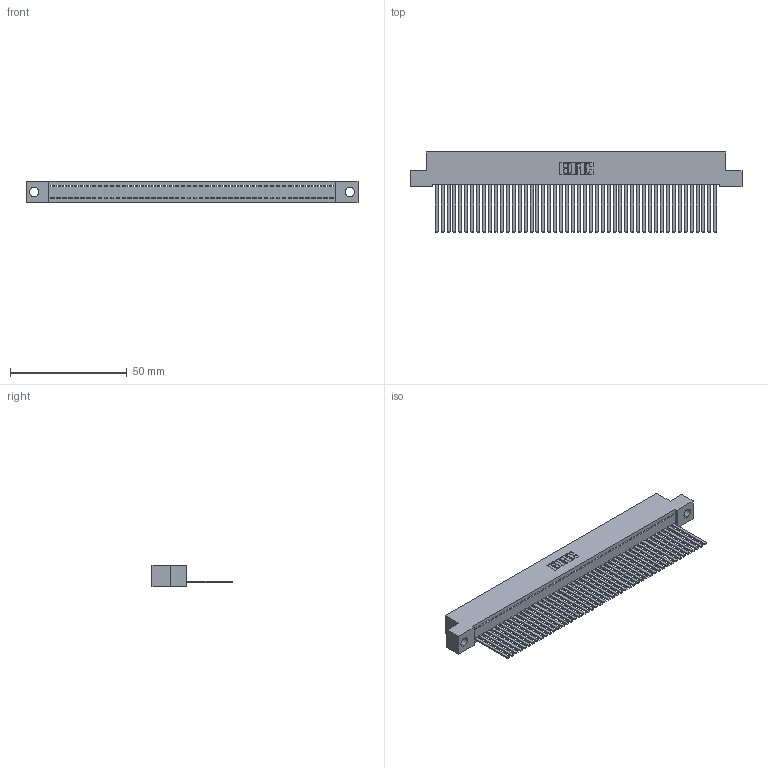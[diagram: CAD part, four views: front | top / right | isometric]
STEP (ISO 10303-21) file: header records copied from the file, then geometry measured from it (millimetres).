
FILE_DESCRIPTION (( 'STEP AP203' ), '1' );
FILE_NAME ('342-048-544-104.STEP', '2018-08-12T18:12:18', ( '' ), ( '' ), 'SwSTEP 2.0', 'SolidWorks 2016', '' );
FILE_SCHEMA (( 'CONFIG_CONTROL_DESIGN' ));
Length unit declared in the file: inch
Products named in the file (3): 342 Part_.156 TH; 345-292-001_345-293-144; 342-048-544-104
Assembly tree (49 placements, depth 2):
  342-048-544-104
    342 Part_.156 TH
    345-292-001_345-293-144  x48
Bounding box: 142.24 x 34.3 x 9.4 mm (x, y, z)
Volume: 12962.6 mm3; surface area: 20547.9 mm2
Topology: 49 solids, 49 shells, 2606 faces, 7883 edges, 5190 vertices
Faces by surface type: plane 1890, cylinder 716
Entity records: 28255 total; most frequent: CARTESIAN_POINT 4878, ORIENTED_EDGE 4862, DIRECTION 4099, EDGE_CURVE 2431, LINE 2307, VECTOR 2307, VERTEX_POINT 1618, AXIS2_PLACEMENT_3D 896
